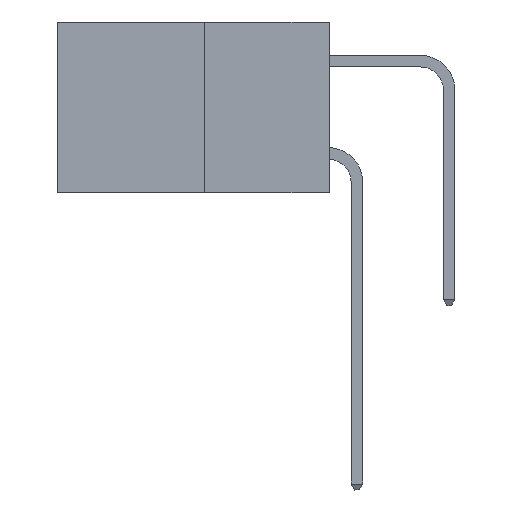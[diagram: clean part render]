
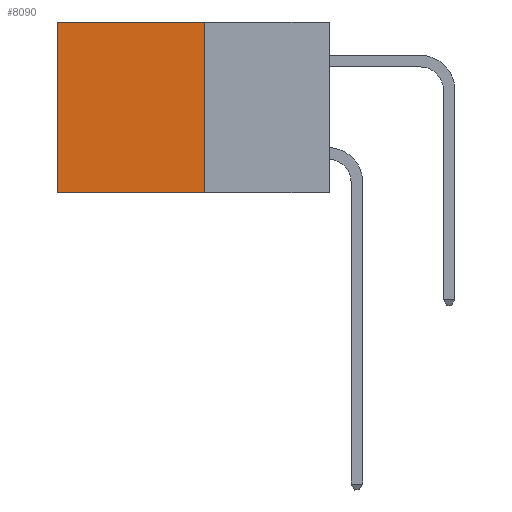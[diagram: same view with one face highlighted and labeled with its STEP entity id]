
A CAD part, left-side view. The second image highlights one B-rep face of the part: STEP entity #8090.
In plain terms, the highlighted planar face has unit normal (-1, 0, 0).
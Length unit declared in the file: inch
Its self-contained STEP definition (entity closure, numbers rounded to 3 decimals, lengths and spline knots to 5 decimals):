
#180 = EDGE_CURVE ( 'NONE', #10513, #4430, #2468, .T. ) ;
#1057 = EDGE_CURVE ( 'NONE', #7397, #12753, #10430, .T. ) ;
#1360 = CARTESIAN_POINT ( 'NONE',  ( 0.277, 0.27, -0.37 ) ) ;
#1448 = CARTESIAN_POINT ( 'NONE',  ( 0.277, 0.59, -0.37 ) ) ;
#2195 = EDGE_CURVE ( 'NONE', #7397, #10513, #7940, .T. ) ;
#2351 = CARTESIAN_POINT ( 'NONE',  ( 0.277, 0.27, 0. ) ) ;
#2468 = LINE ( 'NONE', #1448, #7529 ) ;
#2824 = ORIENTED_EDGE ( 'NONE', *, *, #1057, .F. ) ;
#4430 = VERTEX_POINT ( 'NONE', #12253 ) ;
#4914 = LINE ( 'NONE', #5519, #7275 ) ;
#4940 = VECTOR ( 'NONE', #10464, 39.37008 ) ;
#5286 = AXIS2_PLACEMENT_3D ( 'NONE', #1360, #11372, #5434 ) ;
#5434 = DIRECTION ( 'NONE',  ( 0., 0., -1. ) ) ;
#5519 = CARTESIAN_POINT ( 'NONE',  ( 0.277, 0.27, -0.37 ) ) ;
#5614 = ORIENTED_EDGE ( 'NONE', *, *, #2195, .T. ) ;
#5835 = CARTESIAN_POINT ( 'NONE',  ( 0.277, 0.27, -0.37 ) ) ;
#6515 = DIRECTION ( 'NONE',  ( 0., 1., 0. ) ) ;
#6674 = CARTESIAN_POINT ( 'NONE',  ( 0.277, 0.59, 0. ) ) ;
#7275 = VECTOR ( 'NONE', #6515, 39.37008 ) ;
#7397 = VERTEX_POINT ( 'NONE', #2351 ) ;
#7410 = PLANE ( 'NONE',  #5286 ) ;
#7497 = FACE_OUTER_BOUND ( 'NONE', #7778, .T. ) ;
#7529 = VECTOR ( 'NONE', #10514, 39.37008 ) ;
#7778 = EDGE_LOOP ( 'NONE', ( #8913, #10591, #2824, #5614 ) ) ;
#7827 = VECTOR ( 'NONE', #8841, 39.37008 ) ;
#7940 = LINE ( 'NONE', #9460, #4940 ) ;
#8090 = ADVANCED_FACE ( 'NONE', ( #7497 ), #7410, .F. ) ;
#8841 = DIRECTION ( 'NONE',  ( 0., 0., -1. ) ) ;
#8913 = ORIENTED_EDGE ( 'NONE', *, *, #180, .T. ) ;
#9460 = CARTESIAN_POINT ( 'NONE',  ( 0.277, 0.27, 0. ) ) ;
#10430 = LINE ( 'NONE', #5835, #7827 ) ;
#10464 = DIRECTION ( 'NONE',  ( 0., 1., 0. ) ) ;
#10513 = VERTEX_POINT ( 'NONE', #6674 ) ;
#10514 = DIRECTION ( 'NONE',  ( 0., 0., -1. ) ) ;
#10538 = CARTESIAN_POINT ( 'NONE',  ( 0.277, 0.27, -0.37 ) ) ;
#10591 = ORIENTED_EDGE ( 'NONE', *, *, #11698, .F. ) ;
#11372 = DIRECTION ( 'NONE',  ( 1., 0., 0. ) ) ;
#11698 = EDGE_CURVE ( 'NONE', #12753, #4430, #4914, .T. ) ;
#12253 = CARTESIAN_POINT ( 'NONE',  ( 0.277, 0.59, -0.37 ) ) ;
#12753 = VERTEX_POINT ( 'NONE', #10538 ) ;
